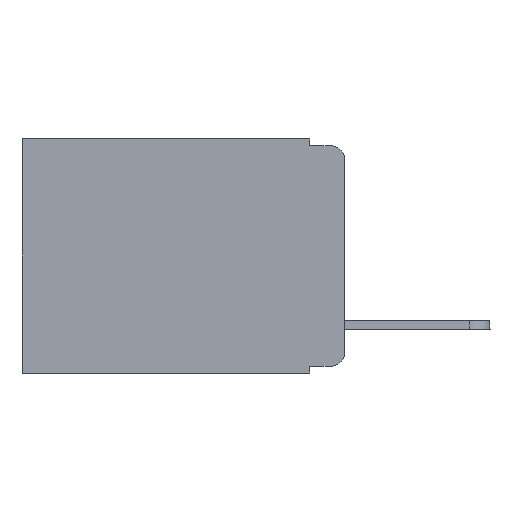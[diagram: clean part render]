
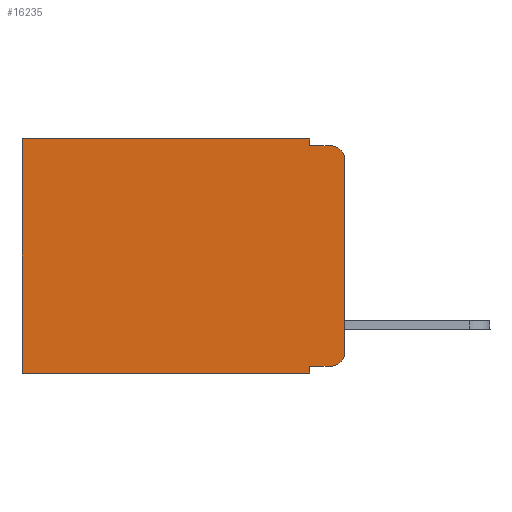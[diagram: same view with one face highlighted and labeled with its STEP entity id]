
A CAD part, left-side view. The second image highlights one B-rep face of the part: STEP entity #16235.
In plain terms, the highlighted planar face has unit normal (-1, 0, 0).
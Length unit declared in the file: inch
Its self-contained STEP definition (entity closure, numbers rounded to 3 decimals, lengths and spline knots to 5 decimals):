
#485 = CARTESIAN_POINT ( 'NONE',  ( 0.298, 0.051, -0.01 ) ) ;
#859 = EDGE_CURVE ( 'NONE', #7682, #18751, #9292, .T. ) ;
#948 = DIRECTION ( 'NONE',  ( 0., 1., 0. ) ) ;
#1168 = CARTESIAN_POINT ( 'NONE',  ( 0.298, 0.051, -0.01 ) ) ;
#1906 = DIRECTION ( 'NONE',  ( 0., -1., 0. ) ) ;
#1988 = CARTESIAN_POINT ( 'NONE',  ( 0.298, 0.02, -0.01 ) ) ;
#2811 = VERTEX_POINT ( 'NONE', #11894 ) ;
#2985 = AXIS2_PLACEMENT_3D ( 'NONE', #12248, #6289, #10464 ) ;
#3465 = ORIENTED_EDGE ( 'NONE', *, *, #16273, .F. ) ;
#3571 = VECTOR ( 'NONE', #12080, 39.37008 ) ;
#3838 = ORIENTED_EDGE ( 'NONE', *, *, #15017, .F. ) ;
#4709 = CIRCLE ( 'NONE', #7861, 0.02 ) ;
#4844 = EDGE_CURVE ( 'NONE', #12311, #18751, #15064, .T. ) ;
#4973 = VERTEX_POINT ( 'NONE', #11348 ) ;
#5394 = EDGE_CURVE ( 'NONE', #15392, #13297, #8666, .T. ) ;
#5472 = AXIS2_PLACEMENT_3D ( 'NONE', #16134, #17435, #15857 ) ;
#5587 = VERTEX_POINT ( 'NONE', #6462 ) ;
#5836 = ORIENTED_EDGE ( 'NONE', *, *, #16043, .T. ) ;
#5878 = CARTESIAN_POINT ( 'NONE',  ( 0.298, 0., -0.313 ) ) ;
#6289 = DIRECTION ( 'NONE',  ( -1., 0., 0. ) ) ;
#6402 = ORIENTED_EDGE ( 'NONE', *, *, #4844, .T. ) ;
#6462 = CARTESIAN_POINT ( 'NONE',  ( 0.298, 0.051, -0.343 ) ) ;
#6493 = LINE ( 'NONE', #16931, #11505 ) ;
#6498 = EDGE_CURVE ( 'NONE', #7682, #13297, #4709, .T. ) ;
#6550 = VECTOR ( 'NONE', #19112, 39.37008 ) ;
#6708 = DIRECTION ( 'NONE',  ( 0., 0., -1. ) ) ;
#6983 = ORIENTED_EDGE ( 'NONE', *, *, #5394, .F. ) ;
#7077 = VECTOR ( 'NONE', #9198, 39.37008 ) ;
#7342 = ORIENTED_EDGE ( 'NONE', *, *, #16598, .T. ) ;
#7682 = VERTEX_POINT ( 'NONE', #16957 ) ;
#7825 = ORIENTED_EDGE ( 'NONE', *, *, #9059, .T. ) ;
#7861 = AXIS2_PLACEMENT_3D ( 'NONE', #12783, #8206, #9886 ) ;
#7883 = VECTOR ( 'NONE', #948, 39.37008 ) ;
#8110 = LINE ( 'NONE', #11378, #8290 ) ;
#8206 = DIRECTION ( 'NONE',  ( -1., 0., 0. ) ) ;
#8290 = VECTOR ( 'NONE', #6708, 39.37008 ) ;
#8312 = CARTESIAN_POINT ( 'NONE',  ( 0.298, 0., 0. ) ) ;
#8381 = ORIENTED_EDGE ( 'NONE', *, *, #6498, .T. ) ;
#8666 = LINE ( 'NONE', #1168, #15946 ) ;
#8722 = CARTESIAN_POINT ( 'NONE',  ( 0.298, 0., -0.343 ) ) ;
#9059 = EDGE_CURVE ( 'NONE', #2811, #10561, #12990, .T. ) ;
#9198 = DIRECTION ( 'NONE',  ( 0., 0., -1. ) ) ;
#9292 = LINE ( 'NONE', #13466, #7077 ) ;
#9886 = DIRECTION ( 'NONE',  ( 0., 0., -1. ) ) ;
#10464 = DIRECTION ( 'NONE',  ( 0., 0., -1. ) ) ;
#10525 = EDGE_LOOP ( 'NONE', ( #13976, #8381, #6983, #3465, #7825, #5836, #17144, #3838, #7342, #6402 ) ) ;
#10561 = VERTEX_POINT ( 'NONE', #18355 ) ;
#11348 = CARTESIAN_POINT ( 'NONE',  ( 0.298, 0.473, -0.343 ) ) ;
#11378 = CARTESIAN_POINT ( 'NONE',  ( 0.298, 0.051, 0. ) ) ;
#11505 = VECTOR ( 'NONE', #1906, 39.37008 ) ;
#11894 = CARTESIAN_POINT ( 'NONE',  ( 0.298, 0.051, 0. ) ) ;
#11934 = EDGE_CURVE ( 'NONE', #5587, #4973, #13011, .T. ) ;
#12080 = DIRECTION ( 'NONE',  ( 0., 0., -1. ) ) ;
#12248 = CARTESIAN_POINT ( 'NONE',  ( 0.298, 0.02, -0.313 ) ) ;
#12262 = VERTEX_POINT ( 'NONE', #14189 ) ;
#12311 = VERTEX_POINT ( 'NONE', #18432 ) ;
#12392 = FACE_OUTER_BOUND ( 'NONE', #10525, .T. ) ;
#12783 = CARTESIAN_POINT ( 'NONE',  ( 0.298, 0.02, -0.03 ) ) ;
#12990 = LINE ( 'NONE', #8312, #6550 ) ;
#13011 = LINE ( 'NONE', #8722, #7883 ) ;
#13297 = VERTEX_POINT ( 'NONE', #1988 ) ;
#13428 = DIRECTION ( 'NONE',  ( 0., -1., 0. ) ) ;
#13466 = CARTESIAN_POINT ( 'NONE',  ( 0.298, 0., 0. ) ) ;
#13976 = ORIENTED_EDGE ( 'NONE', *, *, #859, .F. ) ;
#14189 = CARTESIAN_POINT ( 'NONE',  ( 0.298, 0.051, -0.333 ) ) ;
#15017 = EDGE_CURVE ( 'NONE', #12262, #5587, #8110, .T. ) ;
#15064 = CIRCLE ( 'NONE', #2985, 0.02 ) ;
#15162 = LINE ( 'NONE', #17824, #3571 ) ;
#15392 = VERTEX_POINT ( 'NONE', #485 ) ;
#15760 = DIRECTION ( 'NONE',  ( 0., 0., -1. ) ) ;
#15857 = DIRECTION ( 'NONE',  ( 0., 0., -1. ) ) ;
#15946 = VECTOR ( 'NONE', #13428, 39.37008 ) ;
#16043 = EDGE_CURVE ( 'NONE', #10561, #4973, #15162, .T. ) ;
#16134 = CARTESIAN_POINT ( 'NONE',  ( 0.298, 0., 0. ) ) ;
#16235 = ADVANCED_FACE ( 'NONE', ( #12392 ), #18426, .F. ) ;
#16273 = EDGE_CURVE ( 'NONE', #2811, #15392, #18819, .T. ) ;
#16598 = EDGE_CURVE ( 'NONE', #12262, #12311, #6493, .T. ) ;
#16931 = CARTESIAN_POINT ( 'NONE',  ( 0.298, 0.051, -0.333 ) ) ;
#16957 = CARTESIAN_POINT ( 'NONE',  ( 0.298, 0., -0.03 ) ) ;
#17144 = ORIENTED_EDGE ( 'NONE', *, *, #11934, .F. ) ;
#17435 = DIRECTION ( 'NONE',  ( 1., 0., 0. ) ) ;
#17611 = CARTESIAN_POINT ( 'NONE',  ( 0.298, 0.051, 0. ) ) ;
#17824 = CARTESIAN_POINT ( 'NONE',  ( 0.298, 0.473, 0. ) ) ;
#18355 = CARTESIAN_POINT ( 'NONE',  ( 0.298, 0.473, 0. ) ) ;
#18426 = PLANE ( 'NONE',  #5472 ) ;
#18432 = CARTESIAN_POINT ( 'NONE',  ( 0.298, 0.02, -0.333 ) ) ;
#18751 = VERTEX_POINT ( 'NONE', #5878 ) ;
#18819 = LINE ( 'NONE', #17611, #19085 ) ;
#19085 = VECTOR ( 'NONE', #15760, 39.37008 ) ;
#19112 = DIRECTION ( 'NONE',  ( 0., 1., 0. ) ) ;
